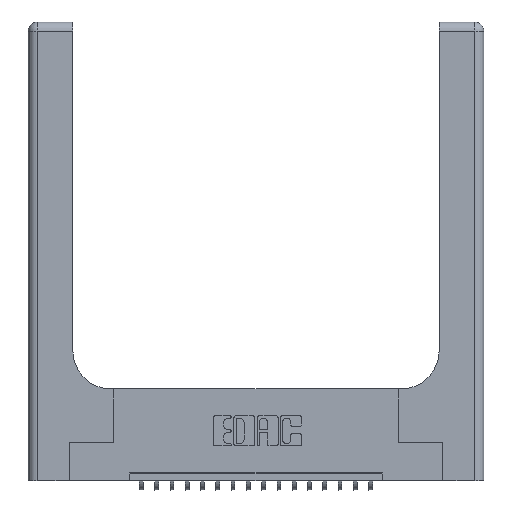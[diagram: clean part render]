
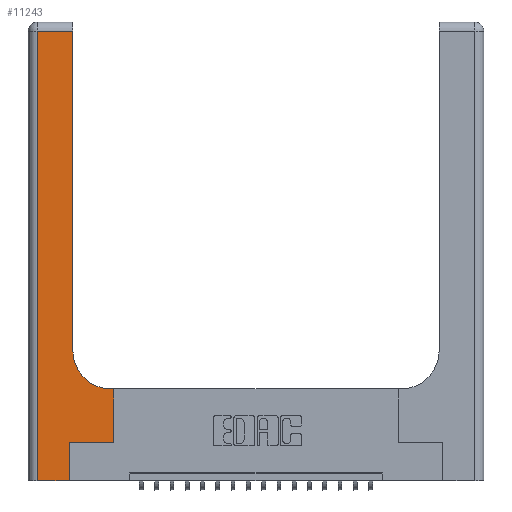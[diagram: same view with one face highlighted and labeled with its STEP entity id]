
A CAD part, top view. The second image highlights one B-rep face of the part: STEP entity #11243.
In plain terms, the highlighted planar face has unit normal (0, 0, 1).
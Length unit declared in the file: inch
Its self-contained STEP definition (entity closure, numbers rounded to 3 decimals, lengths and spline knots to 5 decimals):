
#362 = EDGE_CURVE ( 'NONE', #17658, #13111, #15926, .T. ) ;
#411 = ORIENTED_EDGE ( 'NONE', *, *, #6141, .T. ) ;
#537 = EDGE_CURVE ( 'NONE', #13111, #12684, #7887, .T. ) ;
#979 = DIRECTION ( 'NONE',  ( 0., 1., 0. ) ) ;
#1142 = EDGE_CURVE ( 'NONE', #12684, #18332, #1363, .T. ) ;
#1363 = LINE ( 'NONE', #7385, #20460 ) ;
#1605 = CIRCLE ( 'NONE', #3667, 0.25 ) ;
#1688 = AXIS2_PLACEMENT_3D ( 'NONE', #10298, #7265, #8542 ) ;
#1759 = ORIENTED_EDGE ( 'NONE', *, *, #10712, .T. ) ;
#1835 = CARTESIAN_POINT ( 'NONE',  ( 0.2915, 0.85, 0.37 ) ) ;
#2053 = CARTESIAN_POINT ( 'NONE',  ( 0.5585, 0.25, 0.37 ) ) ;
#2607 = CARTESIAN_POINT ( 'NONE',  ( 0.269, 0., 0.37 ) ) ;
#2799 = ORIENTED_EDGE ( 'NONE', *, *, #537, .T. ) ;
#3399 = DIRECTION ( 'NONE',  ( 0., -1., 0. ) ) ;
#3667 = AXIS2_PLACEMENT_3D ( 'NONE', #16672, #18281, #11898 ) ;
#3768 = CARTESIAN_POINT ( 'NONE',  ( 0., 2.94, 0.37 ) ) ;
#3867 = CARTESIAN_POINT ( 'NONE',  ( 0.06, 0., 0.37 ) ) ;
#3868 = VERTEX_POINT ( 'NONE', #2053 ) ;
#3923 = ORIENTED_EDGE ( 'NONE', *, *, #4418, .T. ) ;
#4418 = EDGE_CURVE ( 'NONE', #16087, #7367, #16084, .T. ) ;
#4764 = ORIENTED_EDGE ( 'NONE', *, *, #1142, .T. ) ;
#4911 = ORIENTED_EDGE ( 'NONE', *, *, #9134, .T. ) ;
#4976 = VECTOR ( 'NONE', #16052, 39.37008 ) ;
#5079 = VECTOR ( 'NONE', #979, 39.37008 ) ;
#5360 = VECTOR ( 'NONE', #17381, 39.37008 ) ;
#6140 = CARTESIAN_POINT ( 'NONE',  ( 0.269, 0.25, 0.37 ) ) ;
#6141 = EDGE_CURVE ( 'NONE', #3868, #16087, #14541, .T. ) ;
#6698 = CARTESIAN_POINT ( 'NONE',  ( 0.5585, 0.25, 0.37 ) ) ;
#7127 = CARTESIAN_POINT ( 'NONE',  ( 0.5415, 0.6, 0.37 ) ) ;
#7265 = DIRECTION ( 'NONE',  ( 0., 0., -1. ) ) ;
#7367 = VERTEX_POINT ( 'NONE', #7127 ) ;
#7385 = CARTESIAN_POINT ( 'NONE',  ( 0.269, 0., 0.37 ) ) ;
#7617 = CARTESIAN_POINT ( 'NONE',  ( 0., 0., 0.37 ) ) ;
#7799 = VECTOR ( 'NONE', #7996, 39.37008 ) ;
#7887 = LINE ( 'NONE', #7617, #17686 ) ;
#7996 = DIRECTION ( 'NONE',  ( -1., 0., 0. ) ) ;
#8475 = VERTEX_POINT ( 'NONE', #1835 ) ;
#8542 = DIRECTION ( 'NONE',  ( -1., 0., 0. ) ) ;
#8804 = PLANE ( 'NONE',  #1688 ) ;
#9134 = EDGE_CURVE ( 'NONE', #18332, #3868, #9146, .T. ) ;
#9146 = LINE ( 'NONE', #6140, #5360 ) ;
#10298 = CARTESIAN_POINT ( 'NONE',  ( 0., 3., 0.37 ) ) ;
#10450 = VECTOR ( 'NONE', #19687, 39.37008 ) ;
#10626 = DIRECTION ( 'NONE',  ( 0., 1., 0. ) ) ;
#10712 = EDGE_CURVE ( 'NONE', #8475, #13737, #19407, .T. ) ;
#11151 = CARTESIAN_POINT ( 'NONE',  ( 0.06, 2.94, 0.37 ) ) ;
#11243 = ADVANCED_FACE ( 'NONE', ( #13371 ), #8804, .F. ) ;
#11294 = CARTESIAN_POINT ( 'NONE',  ( 0.2915, 0.6, 0.37 ) ) ;
#11414 = VECTOR ( 'NONE', #3399, 39.37008 ) ;
#11663 = CARTESIAN_POINT ( 'NONE',  ( 0.06, 3., 0.37 ) ) ;
#11898 = DIRECTION ( 'NONE',  ( 1., 0., 0. ) ) ;
#12684 = VERTEX_POINT ( 'NONE', #2607 ) ;
#13111 = VERTEX_POINT ( 'NONE', #3867 ) ;
#13371 = FACE_OUTER_BOUND ( 'NONE', #14234, .T. ) ;
#13737 = VERTEX_POINT ( 'NONE', #16552 ) ;
#14234 = EDGE_LOOP ( 'NONE', ( #1759, #18636, #16321, #2799, #4764, #4911, #411, #3923, #17206 ) ) ;
#14541 = LINE ( 'NONE', #6698, #4976 ) ;
#14770 = CARTESIAN_POINT ( 'NONE',  ( 0.269, 0.25, 0.37 ) ) ;
#15420 = DIRECTION ( 'NONE',  ( 1., 0., 0. ) ) ;
#15926 = LINE ( 'NONE', #11663, #11414 ) ;
#16052 = DIRECTION ( 'NONE',  ( 0., 1., 0. ) ) ;
#16084 = LINE ( 'NONE', #11294, #7799 ) ;
#16087 = VERTEX_POINT ( 'NONE', #20480 ) ;
#16267 = EDGE_CURVE ( 'NONE', #13737, #17658, #17983, .T. ) ;
#16321 = ORIENTED_EDGE ( 'NONE', *, *, #362, .T. ) ;
#16552 = CARTESIAN_POINT ( 'NONE',  ( 0.2915, 2.94, 0.37 ) ) ;
#16672 = CARTESIAN_POINT ( 'NONE',  ( 0.5415, 0.85, 0.37 ) ) ;
#17206 = ORIENTED_EDGE ( 'NONE', *, *, #17893, .T. ) ;
#17381 = DIRECTION ( 'NONE',  ( 1., 0., 0. ) ) ;
#17658 = VERTEX_POINT ( 'NONE', #11151 ) ;
#17686 = VECTOR ( 'NONE', #15420, 39.37008 ) ;
#17893 = EDGE_CURVE ( 'NONE', #7367, #8475, #1605, .T. ) ;
#17983 = LINE ( 'NONE', #3768, #10450 ) ;
#18281 = DIRECTION ( 'NONE',  ( 0., 0., -1. ) ) ;
#18332 = VERTEX_POINT ( 'NONE', #14770 ) ;
#18636 = ORIENTED_EDGE ( 'NONE', *, *, #16267, .T. ) ;
#19407 = LINE ( 'NONE', #20070, #5079 ) ;
#19687 = DIRECTION ( 'NONE',  ( -1., 0., 0. ) ) ;
#20070 = CARTESIAN_POINT ( 'NONE',  ( 0.2915, 3., 0.37 ) ) ;
#20460 = VECTOR ( 'NONE', #10626, 39.37008 ) ;
#20480 = CARTESIAN_POINT ( 'NONE',  ( 0.5585, 0.6, 0.37 ) ) ;
